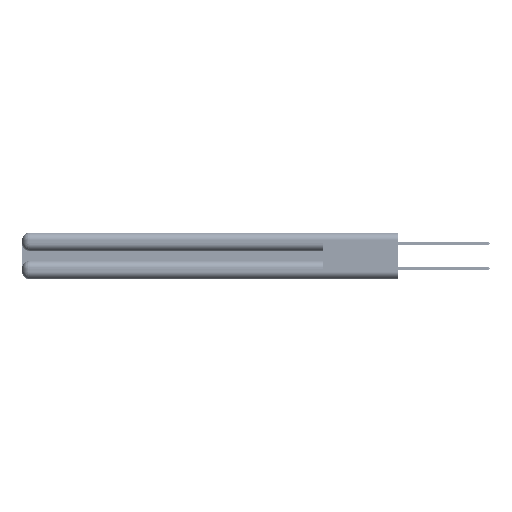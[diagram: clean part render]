
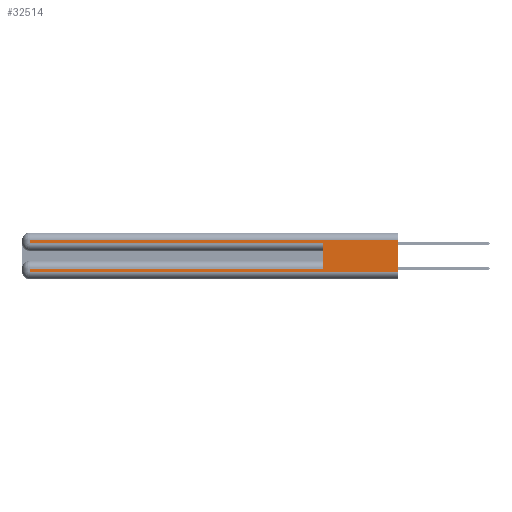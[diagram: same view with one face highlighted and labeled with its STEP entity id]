
A CAD part, left-side view. The second image highlights one B-rep face of the part: STEP entity #32514.
In plain terms, the highlighted planar face has unit normal (-1, 0, 0).
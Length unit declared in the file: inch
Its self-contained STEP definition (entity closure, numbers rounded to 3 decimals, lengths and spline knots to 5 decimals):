
#214 = VECTOR ( 'NONE', #5812, 39.37008 ) ;
#1122 = CARTESIAN_POINT ( 'NONE',  ( 0., 2.94, 0.06 ) ) ;
#1502 = CARTESIAN_POINT ( 'NONE',  ( 0., 0.6, 0.085 ) ) ;
#2652 = LINE ( 'NONE', #14563, #35511 ) ;
#2780 = EDGE_CURVE ( 'NONE', #5299, #48586, #36333, .T. ) ;
#3442 = VECTOR ( 'NONE', #26774, 39.37008 ) ;
#4762 = LINE ( 'NONE', #31272, #3442 ) ;
#5299 = VERTEX_POINT ( 'NONE', #1122 ) ;
#5812 = DIRECTION ( 'NONE',  ( 0., 0., -1. ) ) ;
#6025 = VECTOR ( 'NONE', #14214, 39.37008 ) ;
#6781 = DIRECTION ( 'NONE',  ( 0., 0., -1. ) ) ;
#7230 = VERTEX_POINT ( 'NONE', #1502 ) ;
#7400 = LINE ( 'NONE', #26976, #6025 ) ;
#7648 = LINE ( 'NONE', #14196, #41856 ) ;
#8601 = EDGE_CURVE ( 'NONE', #37077, #26544, #22983, .T. ) ;
#10057 = ORIENTED_EDGE ( 'NONE', *, *, #21310, .T. ) ;
#11399 = LINE ( 'NONE', #32423, #12749 ) ;
#11940 = LINE ( 'NONE', #40624, #33413 ) ;
#12749 = VECTOR ( 'NONE', #6781, 39.37008 ) ;
#14196 = CARTESIAN_POINT ( 'NONE',  ( 0., 0.6, 0.145 ) ) ;
#14214 = DIRECTION ( 'NONE',  ( 0., 0., -1. ) ) ;
#14563 = CARTESIAN_POINT ( 'NONE',  ( 0., 0., 0.285 ) ) ;
#14795 = CARTESIAN_POINT ( 'NONE',  ( 0., 0., 0.31 ) ) ;
#17209 = VERTEX_POINT ( 'NONE', #33826 ) ;
#17671 = FACE_OUTER_BOUND ( 'NONE', #33898, .T. ) ;
#18217 = CARTESIAN_POINT ( 'NONE',  ( 0., 2.94, 0.285 ) ) ;
#20873 = EDGE_CURVE ( 'NONE', #7230, #33844, #4762, .T. ) ;
#21310 = EDGE_CURVE ( 'NONE', #33844, #5299, #11399, .T. ) ;
#22983 = LINE ( 'NONE', #40132, #214 ) ;
#23367 = DIRECTION ( 'NONE',  ( 0., -1., 0. ) ) ;
#24890 = VECTOR ( 'NONE', #23367, 39.37008 ) ;
#25091 = DIRECTION ( 'NONE',  ( 1., 0., 0. ) ) ;
#26544 = VERTEX_POINT ( 'NONE', #18217 ) ;
#26774 = DIRECTION ( 'NONE',  ( 0., 1., 0. ) ) ;
#26976 = CARTESIAN_POINT ( 'NONE',  ( 0., 0., 0.37 ) ) ;
#27187 = ORIENTED_EDGE ( 'NONE', *, *, #44366, .F. ) ;
#27297 = DIRECTION ( 'NONE',  ( 0., -1., 0. ) ) ;
#28098 = CARTESIAN_POINT ( 'NONE',  ( 0., 2.94, 0.31 ) ) ;
#29218 = CARTESIAN_POINT ( 'NONE',  ( 0., 0., 0.37 ) ) ;
#30864 = ORIENTED_EDGE ( 'NONE', *, *, #40764, .T. ) ;
#31272 = CARTESIAN_POINT ( 'NONE',  ( 0., 0., 0.085 ) ) ;
#31332 = AXIS2_PLACEMENT_3D ( 'NONE', #29218, #25091, #55106 ) ;
#32423 = CARTESIAN_POINT ( 'NONE',  ( 0., 2.94, 0.37 ) ) ;
#32514 = ADVANCED_FACE ( 'NONE', ( #17671 ), #50782, .F. ) ;
#33413 = VECTOR ( 'NONE', #44931, 39.37008 ) ;
#33826 = CARTESIAN_POINT ( 'NONE',  ( 0., 0.6, 0.285 ) ) ;
#33844 = VERTEX_POINT ( 'NONE', #50463 ) ;
#33898 = EDGE_LOOP ( 'NONE', ( #44551, #30864, #45155, #47650, #27187, #47413, #10057, #34616 ) ) ;
#34616 = ORIENTED_EDGE ( 'NONE', *, *, #2780, .T. ) ;
#35095 = VERTEX_POINT ( 'NONE', #14795 ) ;
#35511 = VECTOR ( 'NONE', #27297, 39.37008 ) ;
#36333 = LINE ( 'NONE', #53382, #24890 ) ;
#37077 = VERTEX_POINT ( 'NONE', #28098 ) ;
#39939 = EDGE_CURVE ( 'NONE', #26544, #17209, #2652, .T. ) ;
#40132 = CARTESIAN_POINT ( 'NONE',  ( 0., 2.94, 0.37 ) ) ;
#40624 = CARTESIAN_POINT ( 'NONE',  ( 0., 0., 0.31 ) ) ;
#40764 = EDGE_CURVE ( 'NONE', #35095, #37077, #11940, .T. ) ;
#41856 = VECTOR ( 'NONE', #44217, 39.37008 ) ;
#44217 = DIRECTION ( 'NONE',  ( 0., 0., 1. ) ) ;
#44366 = EDGE_CURVE ( 'NONE', #7230, #17209, #7648, .T. ) ;
#44551 = ORIENTED_EDGE ( 'NONE', *, *, #47772, .F. ) ;
#44931 = DIRECTION ( 'NONE',  ( 0., 1., 0. ) ) ;
#45155 = ORIENTED_EDGE ( 'NONE', *, *, #8601, .T. ) ;
#45497 = CARTESIAN_POINT ( 'NONE',  ( 0., 0., 0.06 ) ) ;
#47413 = ORIENTED_EDGE ( 'NONE', *, *, #20873, .T. ) ;
#47650 = ORIENTED_EDGE ( 'NONE', *, *, #39939, .T. ) ;
#47772 = EDGE_CURVE ( 'NONE', #35095, #48586, #7400, .T. ) ;
#48586 = VERTEX_POINT ( 'NONE', #45497 ) ;
#50463 = CARTESIAN_POINT ( 'NONE',  ( 0., 2.94, 0.085 ) ) ;
#50782 = PLANE ( 'NONE',  #31332 ) ;
#53382 = CARTESIAN_POINT ( 'NONE',  ( 0., 0., 0.06 ) ) ;
#55106 = DIRECTION ( 'NONE',  ( 0., 0., -1. ) ) ;
